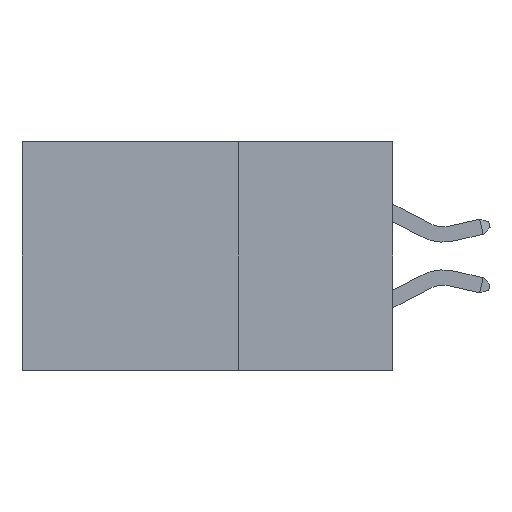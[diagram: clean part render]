
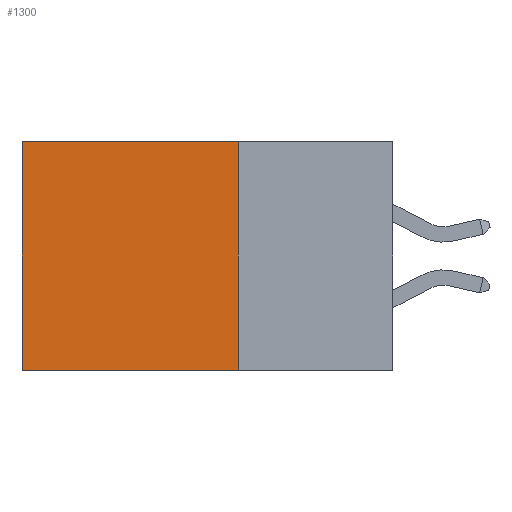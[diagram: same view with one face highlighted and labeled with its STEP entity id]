
A CAD part, left-side view. The second image highlights one B-rep face of the part: STEP entity #1300.
In plain terms, the highlighted planar face has unit normal (-1, 0, 0).
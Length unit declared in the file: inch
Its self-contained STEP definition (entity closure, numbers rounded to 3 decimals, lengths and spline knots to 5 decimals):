
#724 = CARTESIAN_POINT ( 'NONE',  ( 0.2875, 0.6, -0.37 ) ) ;
#919 = AXIS2_PLACEMENT_3D ( 'NONE', #9503, #7247, #6091 ) ;
#1110 = PLANE ( 'NONE',  #919 ) ;
#1182 = CARTESIAN_POINT ( 'NONE',  ( 0.2875, 0.6, 0. ) ) ;
#1300 = ADVANCED_FACE ( 'NONE', ( #12557 ), #1110, .F. ) ;
#1341 = ORIENTED_EDGE ( 'NONE', *, *, #4476, .F. ) ;
#1369 = VECTOR ( 'NONE', #7489, 39.37008 ) ;
#1536 = ORIENTED_EDGE ( 'NONE', *, *, #5684, .F. ) ;
#1763 = LINE ( 'NONE', #12843, #1369 ) ;
#2852 = VERTEX_POINT ( 'NONE', #1182 ) ;
#3546 = DIRECTION ( 'NONE',  ( 0., 0., -1. ) ) ;
#3654 = CARTESIAN_POINT ( 'NONE',  ( 0.2875, 0.25, -0.37 ) ) ;
#3982 = EDGE_LOOP ( 'NONE', ( #6315, #1341, #1536, #5599 ) ) ;
#4476 = EDGE_CURVE ( 'NONE', #7083, #4966, #4625, .T. ) ;
#4625 = LINE ( 'NONE', #4819, #10364 ) ;
#4692 = DIRECTION ( 'NONE',  ( 0., 1., 0. ) ) ;
#4804 = CARTESIAN_POINT ( 'NONE',  ( 0.2875, 0.6, 0. ) ) ;
#4819 = CARTESIAN_POINT ( 'NONE',  ( 0.2875, 0.25, -0.37 ) ) ;
#4966 = VERTEX_POINT ( 'NONE', #724 ) ;
#5599 = ORIENTED_EDGE ( 'NONE', *, *, #12643, .T. ) ;
#5684 = EDGE_CURVE ( 'NONE', #14028, #7083, #9137, .T. ) ;
#5966 = DIRECTION ( 'NONE',  ( 0., 0., -1. ) ) ;
#6024 = VECTOR ( 'NONE', #3546, 39.37008 ) ;
#6091 = DIRECTION ( 'NONE',  ( 0., 0., -1. ) ) ;
#6315 = ORIENTED_EDGE ( 'NONE', *, *, #11515, .T. ) ;
#7000 = CARTESIAN_POINT ( 'NONE',  ( 0.2875, 0.25, 0. ) ) ;
#7083 = VERTEX_POINT ( 'NONE', #3654 ) ;
#7247 = DIRECTION ( 'NONE',  ( 1., 0., 0. ) ) ;
#7257 = VECTOR ( 'NONE', #5966, 39.37008 ) ;
#7489 = DIRECTION ( 'NONE',  ( 0., 1., 0. ) ) ;
#9137 = LINE ( 'NONE', #7000, #6024 ) ;
#9503 = CARTESIAN_POINT ( 'NONE',  ( 0.2875, 0.25, 0. ) ) ;
#10364 = VECTOR ( 'NONE', #4692, 39.37008 ) ;
#11515 = EDGE_CURVE ( 'NONE', #2852, #4966, #13264, .T. ) ;
#12557 = FACE_OUTER_BOUND ( 'NONE', #3982, .T. ) ;
#12643 = EDGE_CURVE ( 'NONE', #14028, #2852, #1763, .T. ) ;
#12843 = CARTESIAN_POINT ( 'NONE',  ( 0.2875, 0.25, 0. ) ) ;
#13199 = CARTESIAN_POINT ( 'NONE',  ( 0.2875, 0.25, 0. ) ) ;
#13264 = LINE ( 'NONE', #4804, #7257 ) ;
#14028 = VERTEX_POINT ( 'NONE', #13199 ) ;
